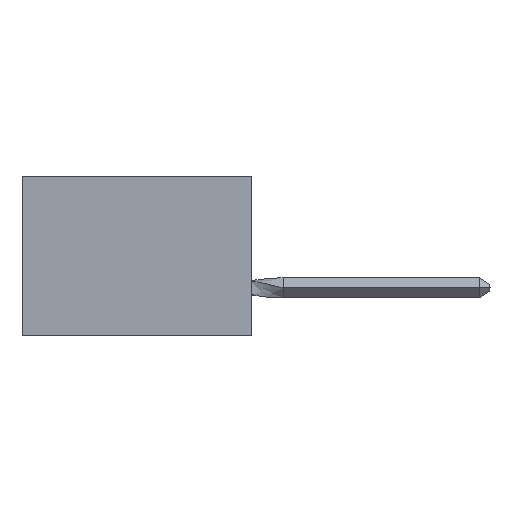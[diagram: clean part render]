
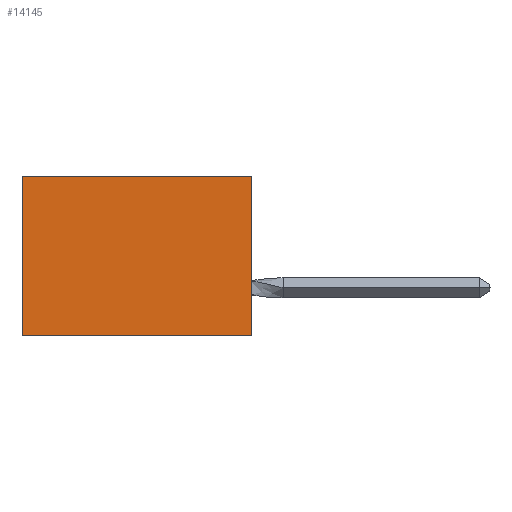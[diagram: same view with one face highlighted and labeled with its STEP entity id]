
A CAD part, left-side view. The second image highlights one B-rep face of the part: STEP entity #14145.
In plain terms, the highlighted planar face has unit normal (-1, 0, 0).
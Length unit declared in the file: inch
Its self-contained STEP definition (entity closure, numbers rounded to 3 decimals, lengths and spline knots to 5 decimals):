
#34 = DIRECTION ( 'NONE',  ( 1., 0., 0. ) ) ;
#240 = VECTOR ( 'NONE', #16924, 39.37008 ) ;
#548 = CARTESIAN_POINT ( 'NONE',  ( 0.305, 0., -0.5 ) ) ;
#1604 = EDGE_CURVE ( 'NONE', #2922, #5182, #9840, .T. ) ;
#2922 = VERTEX_POINT ( 'NONE', #10207 ) ;
#3283 = CARTESIAN_POINT ( 'NONE',  ( 0.305, 0., -0.5 ) ) ;
#3513 = VECTOR ( 'NONE', #15605, 39.37008 ) ;
#4026 = EDGE_CURVE ( 'NONE', #5182, #12316, #8763, .T. ) ;
#4479 = DIRECTION ( 'NONE',  ( 0., 0., -1. ) ) ;
#5048 = ORIENTED_EDGE ( 'NONE', *, *, #1604, .T. ) ;
#5182 = VERTEX_POINT ( 'NONE', #15991 ) ;
#6298 = EDGE_LOOP ( 'NONE', ( #8171, #15855, #21146, #5048 ) ) ;
#6340 = CARTESIAN_POINT ( 'NONE',  ( 0.305, 0.72, -0.5 ) ) ;
#8171 = ORIENTED_EDGE ( 'NONE', *, *, #4026, .T. ) ;
#8763 = LINE ( 'NONE', #6340, #23433 ) ;
#9172 = DIRECTION ( 'NONE',  ( 0., 0., -1. ) ) ;
#9682 = PLANE ( 'NONE',  #20192 ) ;
#9840 = LINE ( 'NONE', #16837, #240 ) ;
#10207 = CARTESIAN_POINT ( 'NONE',  ( 0.305, 0., 0. ) ) ;
#11692 = CARTESIAN_POINT ( 'NONE',  ( 0.305, 0., -0.5 ) ) ;
#12316 = VERTEX_POINT ( 'NONE', #19956 ) ;
#13104 = LINE ( 'NONE', #14677, #17878 ) ;
#14145 = ADVANCED_FACE ( 'NONE', ( #18278 ), #9682, .F. ) ;
#14677 = CARTESIAN_POINT ( 'NONE',  ( 0.305, 0., -0.5 ) ) ;
#15605 = DIRECTION ( 'NONE',  ( 0., 1., 0. ) ) ;
#15855 = ORIENTED_EDGE ( 'NONE', *, *, #17784, .F. ) ;
#15991 = CARTESIAN_POINT ( 'NONE',  ( 0.305, 0.72, 0. ) ) ;
#16837 = CARTESIAN_POINT ( 'NONE',  ( 0.305, 0., 0. ) ) ;
#16924 = DIRECTION ( 'NONE',  ( 0., 1., 0. ) ) ;
#17314 = LINE ( 'NONE', #548, #3513 ) ;
#17433 = DIRECTION ( 'NONE',  ( 0., 0., -1. ) ) ;
#17784 = EDGE_CURVE ( 'NONE', #20058, #12316, #17314, .T. ) ;
#17878 = VECTOR ( 'NONE', #9172, 39.37008 ) ;
#18278 = FACE_OUTER_BOUND ( 'NONE', #6298, .T. ) ;
#18735 = EDGE_CURVE ( 'NONE', #2922, #20058, #13104, .T. ) ;
#19956 = CARTESIAN_POINT ( 'NONE',  ( 0.305, 0.72, -0.5 ) ) ;
#20058 = VERTEX_POINT ( 'NONE', #3283 ) ;
#20192 = AXIS2_PLACEMENT_3D ( 'NONE', #11692, #34, #17433 ) ;
#21146 = ORIENTED_EDGE ( 'NONE', *, *, #18735, .F. ) ;
#23433 = VECTOR ( 'NONE', #4479, 39.37008 ) ;
